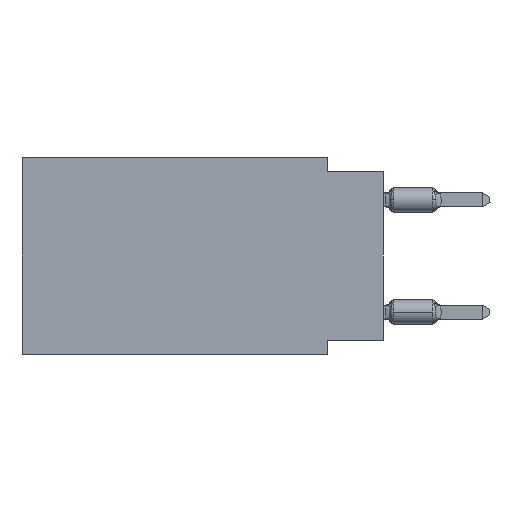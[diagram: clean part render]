
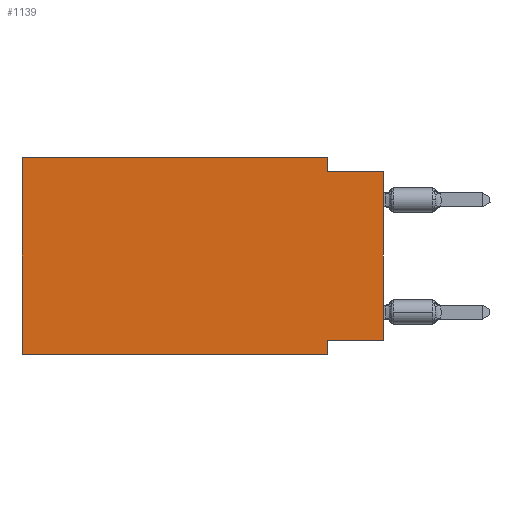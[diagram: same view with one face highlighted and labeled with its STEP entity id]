
A CAD part, left-side view. The second image highlights one B-rep face of the part: STEP entity #1139.
In plain terms, the highlighted planar face has unit normal (-1, 0, 0).
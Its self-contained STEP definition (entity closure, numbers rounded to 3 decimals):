
#466 = EDGE_CURVE ( 'NONE', #20491, #16709, #19249, .T. ) ;
#1032 = DIRECTION ( 'NONE',  ( 0., -1., 0. ) ) ;
#1139 = ADVANCED_FACE ( 'NONE', ( #25491 ), #4634, .F. ) ;
#1182 = ORIENTED_EDGE ( 'NONE', *, *, #18246, .F. ) ;
#1335 = DIRECTION ( 'NONE',  ( 0., 0., -1. ) ) ;
#1576 = VECTOR ( 'NONE', #1032, 1000. ) ;
#1644 = VECTOR ( 'NONE', #32350, 1000. ) ;
#2277 = CARTESIAN_POINT ( 'NONE',  ( 0., 16.383, -8.89 ) ) ;
#2645 = VERTEX_POINT ( 'NONE', #33093 ) ;
#4634 = PLANE ( 'NONE',  #6565 ) ;
#5150 = ORIENTED_EDGE ( 'NONE', *, *, #23289, .T. ) ;
#5218 = VECTOR ( 'NONE', #11153, 1000. ) ;
#5912 = VERTEX_POINT ( 'NONE', #33974 ) ;
#5968 = CARTESIAN_POINT ( 'NONE',  ( 0., 0., 0. ) ) ;
#5995 = VECTOR ( 'NONE', #20056, 1000. ) ;
#6030 = VERTEX_POINT ( 'NONE', #29238 ) ;
#6447 = VERTEX_POINT ( 'NONE', #35284 ) ;
#6565 = AXIS2_PLACEMENT_3D ( 'NONE', #31394, #16442, #16648 ) ;
#6946 = CARTESIAN_POINT ( 'NONE',  ( 0., 16.383, 0. ) ) ;
#7635 = LINE ( 'NONE', #10794, #32220 ) ;
#8056 = CARTESIAN_POINT ( 'NONE',  ( 0., 0., -0.635 ) ) ;
#8125 = VECTOR ( 'NONE', #9698, 1000. ) ;
#8170 = CARTESIAN_POINT ( 'NONE',  ( 0., 16.383, -8.89 ) ) ;
#9698 = DIRECTION ( 'NONE',  ( 0., 0., -1. ) ) ;
#10794 = CARTESIAN_POINT ( 'NONE',  ( 0., 2.54, -8.89 ) ) ;
#11153 = DIRECTION ( 'NONE',  ( 0., -1., 0. ) ) ;
#11736 = CARTESIAN_POINT ( 'NONE',  ( 0., 2.54, -8.255 ) ) ;
#12270 = VERTEX_POINT ( 'NONE', #11736 ) ;
#12703 = ORIENTED_EDGE ( 'NONE', *, *, #14523, .F. ) ;
#12850 = LINE ( 'NONE', #6946, #1576 ) ;
#13347 = CARTESIAN_POINT ( 'NONE',  ( 0., 16.383, 0. ) ) ;
#13727 = ORIENTED_EDGE ( 'NONE', *, *, #466, .F. ) ;
#14049 = EDGE_CURVE ( 'NONE', #16709, #38004, #12850, .T. ) ;
#14523 = EDGE_CURVE ( 'NONE', #6447, #6030, #17109, .T. ) ;
#15786 = CARTESIAN_POINT ( 'NONE',  ( 0., 2.54, 0. ) ) ;
#16442 = DIRECTION ( 'NONE',  ( 1., 0., 0. ) ) ;
#16648 = DIRECTION ( 'NONE',  ( 0., 0., -1. ) ) ;
#16709 = VERTEX_POINT ( 'NONE', #37084 ) ;
#17109 = LINE ( 'NONE', #8056, #5995 ) ;
#18246 = EDGE_CURVE ( 'NONE', #12270, #5912, #7635, .T. ) ;
#18763 = EDGE_CURVE ( 'NONE', #20491, #5912, #38264, .T. ) ;
#19249 = LINE ( 'NONE', #13347, #27890 ) ;
#20056 = DIRECTION ( 'NONE',  ( 0., -1., 0. ) ) ;
#20491 = VERTEX_POINT ( 'NONE', #8170 ) ;
#23289 = EDGE_CURVE ( 'NONE', #2645, #6030, #24044, .T. ) ;
#24044 = LINE ( 'NONE', #5968, #1644 ) ;
#25205 = EDGE_LOOP ( 'NONE', ( #5150, #12703, #35661, #27752, #13727, #33840, #1182, #35043 ) ) ;
#25491 = FACE_OUTER_BOUND ( 'NONE', #25205, .T. ) ;
#26382 = CARTESIAN_POINT ( 'NONE',  ( 0., 0., -8.255 ) ) ;
#27752 = ORIENTED_EDGE ( 'NONE', *, *, #14049, .F. ) ;
#27890 = VECTOR ( 'NONE', #30859, 1000. ) ;
#29238 = CARTESIAN_POINT ( 'NONE',  ( 0., 0., -0.635 ) ) ;
#29297 = CARTESIAN_POINT ( 'NONE',  ( 0., 2.54, 0. ) ) ;
#29922 = LINE ( 'NONE', #26382, #36387 ) ;
#30859 = DIRECTION ( 'NONE',  ( 0., 0., 1. ) ) ;
#30928 = LINE ( 'NONE', #15786, #8125 ) ;
#31394 = CARTESIAN_POINT ( 'NONE',  ( 0., 16.383, 0. ) ) ;
#32220 = VECTOR ( 'NONE', #1335, 1000. ) ;
#32350 = DIRECTION ( 'NONE',  ( 0., 0., 1. ) ) ;
#33093 = CARTESIAN_POINT ( 'NONE',  ( 0., 0., -8.255 ) ) ;
#33840 = ORIENTED_EDGE ( 'NONE', *, *, #18763, .T. ) ;
#33974 = CARTESIAN_POINT ( 'NONE',  ( 0., 2.54, -8.89 ) ) ;
#35043 = ORIENTED_EDGE ( 'NONE', *, *, #36329, .F. ) ;
#35284 = CARTESIAN_POINT ( 'NONE',  ( 0., 2.54, -0.635 ) ) ;
#35618 = DIRECTION ( 'NONE',  ( 0., 1., 0. ) ) ;
#35661 = ORIENTED_EDGE ( 'NONE', *, *, #36137, .F. ) ;
#36137 = EDGE_CURVE ( 'NONE', #38004, #6447, #30928, .T. ) ;
#36329 = EDGE_CURVE ( 'NONE', #2645, #12270, #29922, .T. ) ;
#36387 = VECTOR ( 'NONE', #35618, 1000. ) ;
#37084 = CARTESIAN_POINT ( 'NONE',  ( 0., 16.383, 0. ) ) ;
#38004 = VERTEX_POINT ( 'NONE', #29297 ) ;
#38264 = LINE ( 'NONE', #2277, #5218 ) ;
